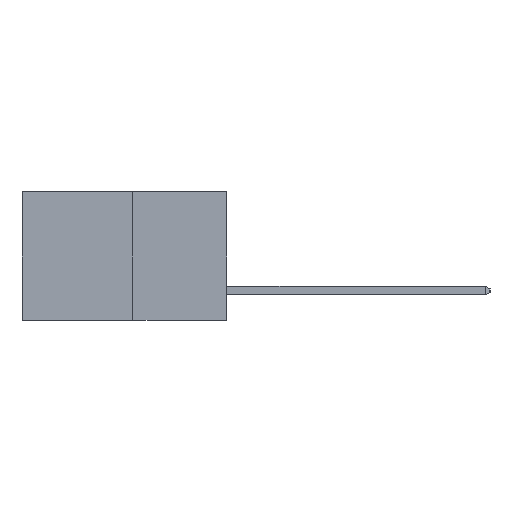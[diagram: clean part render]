
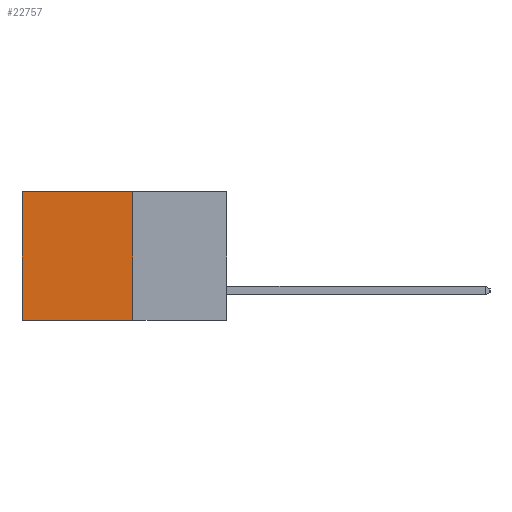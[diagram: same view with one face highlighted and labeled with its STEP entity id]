
A CAD part, left-side view. The second image highlights one B-rep face of the part: STEP entity #22757.
In plain terms, the highlighted planar face has unit normal (-1, 0, 0).
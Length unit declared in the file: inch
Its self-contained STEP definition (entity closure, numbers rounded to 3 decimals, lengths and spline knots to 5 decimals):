
#716 = CARTESIAN_POINT ( 'NONE',  ( 0.277, 0.27, -0.37 ) ) ;
#1028 = AXIS2_PLACEMENT_3D ( 'NONE', #1664, #3855, #18969 ) ;
#1323 = CARTESIAN_POINT ( 'NONE',  ( 0.277, 0.59, -0.37 ) ) ;
#1664 = CARTESIAN_POINT ( 'NONE',  ( 0.277, 0.27, -0.37 ) ) ;
#1895 = VECTOR ( 'NONE', #13819, 39.37008 ) ;
#2092 = VECTOR ( 'NONE', #18052, 39.37008 ) ;
#3205 = CARTESIAN_POINT ( 'NONE',  ( 0.277, 0.59, 0. ) ) ;
#3855 = DIRECTION ( 'NONE',  ( 1., 0., 0. ) ) ;
#4835 = CARTESIAN_POINT ( 'NONE',  ( 0.277, 0.59, -0.37 ) ) ;
#4853 = VERTEX_POINT ( 'NONE', #22691 ) ;
#5732 = DIRECTION ( 'NONE',  ( 0., 0., -1. ) ) ;
#6961 = LINE ( 'NONE', #1323, #23434 ) ;
#7763 = VERTEX_POINT ( 'NONE', #8414 ) ;
#7841 = VERTEX_POINT ( 'NONE', #3205 ) ;
#7902 = LINE ( 'NONE', #716, #2092 ) ;
#8414 = CARTESIAN_POINT ( 'NONE',  ( 0.277, 0.27, -0.37 ) ) ;
#8502 = ORIENTED_EDGE ( 'NONE', *, *, #16467, .T. ) ;
#11647 = CARTESIAN_POINT ( 'NONE',  ( 0.277, 0.27, 0. ) ) ;
#12871 = VECTOR ( 'NONE', #5732, 39.37008 ) ;
#13118 = ORIENTED_EDGE ( 'NONE', *, *, #15613, .T. ) ;
#13545 = LINE ( 'NONE', #22947, #12871 ) ;
#13621 = EDGE_CURVE ( 'NONE', #4853, #7763, #13545, .T. ) ;
#13819 = DIRECTION ( 'NONE',  ( 0., 1., 0. ) ) ;
#14363 = ORIENTED_EDGE ( 'NONE', *, *, #17898, .F. ) ;
#15613 = EDGE_CURVE ( 'NONE', #4853, #7841, #18502, .T. ) ;
#16467 = EDGE_CURVE ( 'NONE', #7841, #22380, #6961, .T. ) ;
#16503 = DIRECTION ( 'NONE',  ( 0., 0., -1. ) ) ;
#16843 = PLANE ( 'NONE',  #1028 ) ;
#17898 = EDGE_CURVE ( 'NONE', #7763, #22380, #7902, .T. ) ;
#18052 = DIRECTION ( 'NONE',  ( 0., 1., 0. ) ) ;
#18502 = LINE ( 'NONE', #11647, #1895 ) ;
#18602 = ORIENTED_EDGE ( 'NONE', *, *, #13621, .F. ) ;
#18969 = DIRECTION ( 'NONE',  ( 0., 0., -1. ) ) ;
#22380 = VERTEX_POINT ( 'NONE', #4835 ) ;
#22691 = CARTESIAN_POINT ( 'NONE',  ( 0.277, 0.27, 0. ) ) ;
#22757 = ADVANCED_FACE ( 'NONE', ( #26199 ), #16843, .F. ) ;
#22947 = CARTESIAN_POINT ( 'NONE',  ( 0.277, 0.27, -0.37 ) ) ;
#22978 = EDGE_LOOP ( 'NONE', ( #8502, #14363, #18602, #13118 ) ) ;
#23434 = VECTOR ( 'NONE', #16503, 39.37008 ) ;
#26199 = FACE_OUTER_BOUND ( 'NONE', #22978, .T. ) ;
